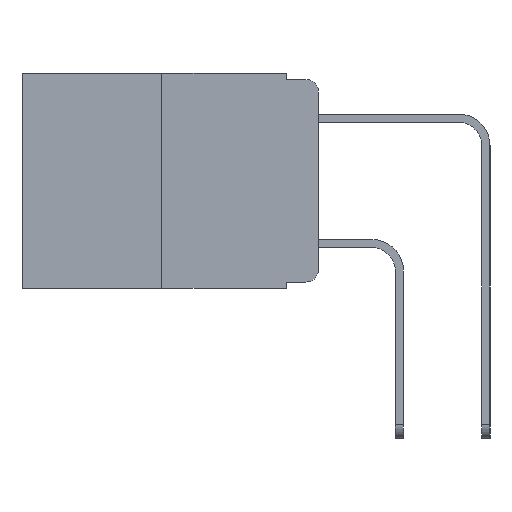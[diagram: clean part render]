
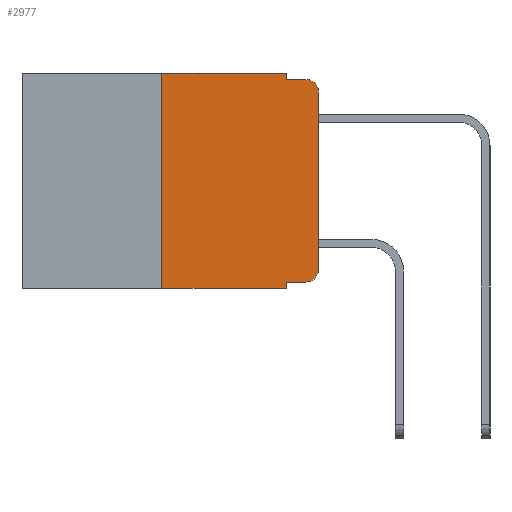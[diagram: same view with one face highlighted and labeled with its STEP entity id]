
A CAD part, left-side view. The second image highlights one B-rep face of the part: STEP entity #2977.
In plain terms, the highlighted planar face has unit normal (-1, 0, 0).
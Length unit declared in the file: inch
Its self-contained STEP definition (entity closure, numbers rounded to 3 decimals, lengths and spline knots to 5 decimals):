
#520 = VECTOR ( 'NONE', #18201, 39.37008 ) ;
#787 = EDGE_CURVE ( 'NONE', #11468, #4452, #1598, .T. ) ;
#956 = EDGE_CURVE ( 'NONE', #14662, #9918, #18948, .T. ) ;
#1302 = DIRECTION ( 'NONE',  ( 0., 0., 1. ) ) ;
#1311 = CARTESIAN_POINT ( 'NONE',  ( 0., 0.051, -0.333 ) ) ;
#1358 = CARTESIAN_POINT ( 'NONE',  ( 0., 0.25, 0. ) ) ;
#1521 = ORIENTED_EDGE ( 'NONE', *, *, #1917, .F. ) ;
#1598 = LINE ( 'NONE', #18150, #520 ) ;
#1917 = EDGE_CURVE ( 'NONE', #1998, #14662, #12238, .T. ) ;
#1998 = VERTEX_POINT ( 'NONE', #18538 ) ;
#2177 = VERTEX_POINT ( 'NONE', #12431 ) ;
#2318 = ORIENTED_EDGE ( 'NONE', *, *, #6491, .F. ) ;
#2395 = ORIENTED_EDGE ( 'NONE', *, *, #13035, .T. ) ;
#2712 = DIRECTION ( 'NONE',  ( -1., 0., 0. ) ) ;
#2732 = VECTOR ( 'NONE', #19299, 39.37008 ) ;
#2977 = ADVANCED_FACE ( 'NONE', ( #14847 ), #15973, .F. ) ;
#3060 = VERTEX_POINT ( 'NONE', #13029 ) ;
#3123 = VERTEX_POINT ( 'NONE', #10071 ) ;
#3192 = EDGE_LOOP ( 'NONE', ( #2395, #11075, #2318, #9004, #18462, #1521, #15229, #14466, #10371, #5143 ) ) ;
#3422 = CARTESIAN_POINT ( 'NONE',  ( 0., 0.051, 0. ) ) ;
#4196 = EDGE_CURVE ( 'NONE', #9918, #7023, #9685, .T. ) ;
#4452 = VERTEX_POINT ( 'NONE', #20756 ) ;
#4653 = LINE ( 'NONE', #17737, #16498 ) ;
#5121 = CIRCLE ( 'NONE', #15597, 0.02 ) ;
#5143 = ORIENTED_EDGE ( 'NONE', *, *, #17500, .T. ) ;
#5303 = VERTEX_POINT ( 'NONE', #9126 ) ;
#6491 = EDGE_CURVE ( 'NONE', #7023, #3123, #4653, .T. ) ;
#7023 = VERTEX_POINT ( 'NONE', #12859 ) ;
#7139 = CARTESIAN_POINT ( 'NONE',  ( 0., 0.25, 0. ) ) ;
#7919 = CARTESIAN_POINT ( 'NONE',  ( 0., 0., 0. ) ) ;
#7973 = DIRECTION ( 'NONE',  ( 0., -1., 0. ) ) ;
#8025 = LINE ( 'NONE', #17389, #9087 ) ;
#8114 = DIRECTION ( 'NONE',  ( 0., 0., -1. ) ) ;
#8391 = DIRECTION ( 'NONE',  ( 0., -1., 0. ) ) ;
#8430 = CARTESIAN_POINT ( 'NONE',  ( 0., 0.051, -0.333 ) ) ;
#8746 = EDGE_CURVE ( 'NONE', #2177, #3123, #13082, .T. ) ;
#9004 = ORIENTED_EDGE ( 'NONE', *, *, #4196, .F. ) ;
#9022 = DIRECTION ( 'NONE',  ( -1., 0., 0. ) ) ;
#9036 = EDGE_CURVE ( 'NONE', #1998, #4452, #8025, .T. ) ;
#9087 = VECTOR ( 'NONE', #7973, 39.37008 ) ;
#9126 = CARTESIAN_POINT ( 'NONE',  ( 0., 0., -0.313 ) ) ;
#9685 = LINE ( 'NONE', #11008, #11678 ) ;
#9712 = CARTESIAN_POINT ( 'NONE',  ( 0., 0.473, 0. ) ) ;
#9918 = VERTEX_POINT ( 'NONE', #3422 ) ;
#10071 = CARTESIAN_POINT ( 'NONE',  ( 0., 0.02, -0.01 ) ) ;
#10371 = ORIENTED_EDGE ( 'NONE', *, *, #19524, .T. ) ;
#11008 = CARTESIAN_POINT ( 'NONE',  ( 0., 0.051, 0. ) ) ;
#11075 = ORIENTED_EDGE ( 'NONE', *, *, #8746, .T. ) ;
#11468 = VERTEX_POINT ( 'NONE', #1311 ) ;
#11678 = VECTOR ( 'NONE', #12573, 39.37008 ) ;
#11739 = VECTOR ( 'NONE', #1302, 39.37008 ) ;
#11842 = DIRECTION ( 'NONE',  ( 0., -1., 0. ) ) ;
#12238 = LINE ( 'NONE', #1358, #11739 ) ;
#12431 = CARTESIAN_POINT ( 'NONE',  ( 0., 0., -0.03 ) ) ;
#12573 = DIRECTION ( 'NONE',  ( 0., 0., -1. ) ) ;
#12642 = CARTESIAN_POINT ( 'NONE',  ( 0., 0.02, -0.313 ) ) ;
#12859 = CARTESIAN_POINT ( 'NONE',  ( 0., 0.051, -0.01 ) ) ;
#13029 = CARTESIAN_POINT ( 'NONE',  ( 0., 0.02, -0.333 ) ) ;
#13035 = EDGE_CURVE ( 'NONE', #5303, #2177, #19933, .T. ) ;
#13082 = CIRCLE ( 'NONE', #18514, 0.02 ) ;
#14200 = DIRECTION ( 'NONE',  ( 0., 0., -1. ) ) ;
#14466 = ORIENTED_EDGE ( 'NONE', *, *, #787, .F. ) ;
#14662 = VERTEX_POINT ( 'NONE', #7139 ) ;
#14847 = FACE_OUTER_BOUND ( 'NONE', #3192, .T. ) ;
#15229 = ORIENTED_EDGE ( 'NONE', *, *, #9036, .T. ) ;
#15597 = AXIS2_PLACEMENT_3D ( 'NONE', #12642, #2712, #14200 ) ;
#15872 = VECTOR ( 'NONE', #11842, 39.37008 ) ;
#15897 = VECTOR ( 'NONE', #20440, 39.37008 ) ;
#15973 = PLANE ( 'NONE',  #17817 ) ;
#16498 = VECTOR ( 'NONE', #8391, 39.37008 ) ;
#17389 = CARTESIAN_POINT ( 'NONE',  ( 0., 0.473, -0.343 ) ) ;
#17495 = DIRECTION ( 'NONE',  ( 1., 0., 0. ) ) ;
#17500 = EDGE_CURVE ( 'NONE', #3060, #5303, #5121, .T. ) ;
#17737 = CARTESIAN_POINT ( 'NONE',  ( 0., 0.051, -0.01 ) ) ;
#17817 = AXIS2_PLACEMENT_3D ( 'NONE', #9712, #17495, #8114 ) ;
#18150 = CARTESIAN_POINT ( 'NONE',  ( 0., 0.051, 0. ) ) ;
#18201 = DIRECTION ( 'NONE',  ( 0., 0., -1. ) ) ;
#18309 = CARTESIAN_POINT ( 'NONE',  ( 0., 0.02, -0.03 ) ) ;
#18462 = ORIENTED_EDGE ( 'NONE', *, *, #956, .F. ) ;
#18514 = AXIS2_PLACEMENT_3D ( 'NONE', #18309, #9022, #19841 ) ;
#18538 = CARTESIAN_POINT ( 'NONE',  ( 0., 0.25, -0.343 ) ) ;
#18948 = LINE ( 'NONE', #20798, #15872 ) ;
#19299 = DIRECTION ( 'NONE',  ( 0., -1., 0. ) ) ;
#19524 = EDGE_CURVE ( 'NONE', #11468, #3060, #20213, .T. ) ;
#19841 = DIRECTION ( 'NONE',  ( 0., 0., -1. ) ) ;
#19933 = LINE ( 'NONE', #7919, #15897 ) ;
#20213 = LINE ( 'NONE', #8430, #2732 ) ;
#20440 = DIRECTION ( 'NONE',  ( 0., 0., 1. ) ) ;
#20756 = CARTESIAN_POINT ( 'NONE',  ( 0., 0.051, -0.343 ) ) ;
#20798 = CARTESIAN_POINT ( 'NONE',  ( 0., 0.473, 0. ) ) ;
